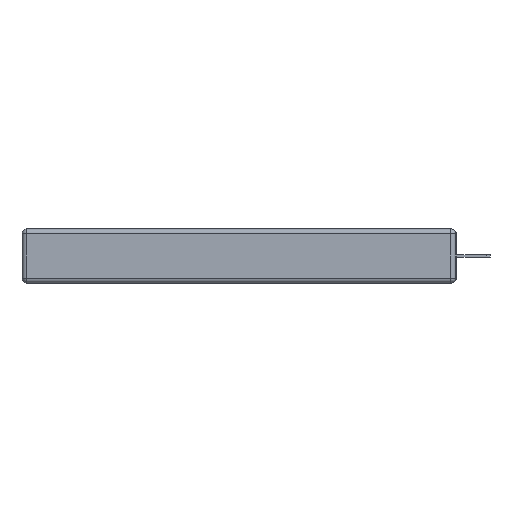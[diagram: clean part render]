
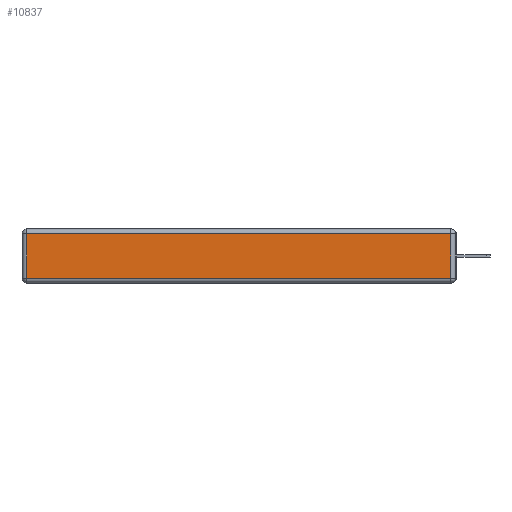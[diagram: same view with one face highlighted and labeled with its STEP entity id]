
A CAD part, left-side view. The second image highlights one B-rep face of the part: STEP entity #10837.
In plain terms, the highlighted planar face has unit normal (-1, 0, 0).
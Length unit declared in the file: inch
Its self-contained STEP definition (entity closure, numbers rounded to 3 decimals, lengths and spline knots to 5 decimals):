
#278 = VERTEX_POINT ( 'NONE', #4204 ) ;
#422 = CARTESIAN_POINT ( 'NONE',  ( 0., 0., -0.343 ) ) ;
#634 = VECTOR ( 'NONE', #3186, 39.37008 ) ;
#689 = DIRECTION ( 'NONE',  ( 0., 0., -1. ) ) ;
#1837 = EDGE_CURVE ( 'NONE', #3921, #3036, #4891, .T. ) ;
#2079 = LINE ( 'NONE', #14035, #7830 ) ;
#2580 = LINE ( 'NONE', #5076, #5310 ) ;
#2764 = DIRECTION ( 'NONE',  ( -1., 0., 0. ) ) ;
#3036 = VERTEX_POINT ( 'NONE', #12596 ) ;
#3186 = DIRECTION ( 'NONE',  ( 0., 0., 1. ) ) ;
#3733 = LINE ( 'NONE', #5489, #634 ) ;
#3877 = PLANE ( 'NONE',  #7802 ) ;
#3893 = DIRECTION ( 'NONE',  ( 0., -1., 0. ) ) ;
#3921 = VERTEX_POINT ( 'NONE', #12893 ) ;
#3948 = FACE_OUTER_BOUND ( 'NONE', #9890, .T. ) ;
#4204 = CARTESIAN_POINT ( 'NONE',  ( 0., 0.03, -0.313 ) ) ;
#4450 = VERTEX_POINT ( 'NONE', #10518 ) ;
#4527 = ORIENTED_EDGE ( 'NONE', *, *, #1837, .T. ) ;
#4891 = LINE ( 'NONE', #9633, #10491 ) ;
#5076 = CARTESIAN_POINT ( 'NONE',  ( 0., 0., -0.313 ) ) ;
#5310 = VECTOR ( 'NONE', #3893, 39.37008 ) ;
#5489 = CARTESIAN_POINT ( 'NONE',  ( 0., 0.03, -0.343 ) ) ;
#5736 = EDGE_CURVE ( 'NONE', #4450, #3921, #2079, .T. ) ;
#6371 = DIRECTION ( 'NONE',  ( 0., 1., 0. ) ) ;
#6487 = EDGE_CURVE ( 'NONE', #278, #4450, #3733, .T. ) ;
#7802 = AXIS2_PLACEMENT_3D ( 'NONE', #422, #2764, #10666 ) ;
#7830 = VECTOR ( 'NONE', #6371, 39.37008 ) ;
#8745 = EDGE_CURVE ( 'NONE', #3036, #278, #2580, .T. ) ;
#9633 = CARTESIAN_POINT ( 'NONE',  ( 0., 2.72, -0.343 ) ) ;
#9890 = EDGE_LOOP ( 'NONE', ( #12744, #12591, #10135, #4527 ) ) ;
#10135 = ORIENTED_EDGE ( 'NONE', *, *, #5736, .T. ) ;
#10491 = VECTOR ( 'NONE', #689, 39.37008 ) ;
#10518 = CARTESIAN_POINT ( 'NONE',  ( 0., 0.03, -0.03 ) ) ;
#10666 = DIRECTION ( 'NONE',  ( 0., 0., 1. ) ) ;
#10837 = ADVANCED_FACE ( 'NONE', ( #3948 ), #3877, .T. ) ;
#12591 = ORIENTED_EDGE ( 'NONE', *, *, #6487, .T. ) ;
#12596 = CARTESIAN_POINT ( 'NONE',  ( 0., 2.72, -0.313 ) ) ;
#12744 = ORIENTED_EDGE ( 'NONE', *, *, #8745, .T. ) ;
#12893 = CARTESIAN_POINT ( 'NONE',  ( 0., 2.72, -0.03 ) ) ;
#14035 = CARTESIAN_POINT ( 'NONE',  ( 0., 2.75, -0.03 ) ) ;
